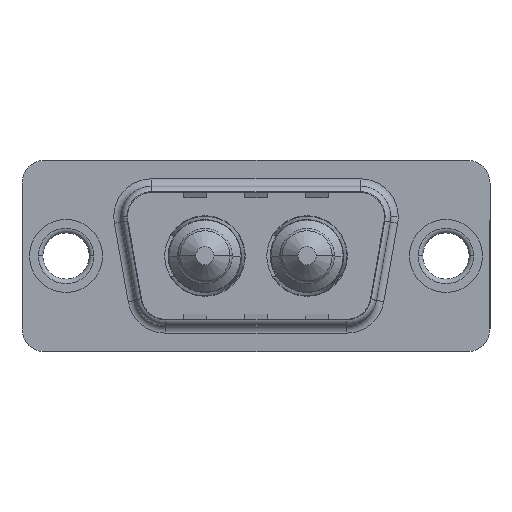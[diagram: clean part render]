
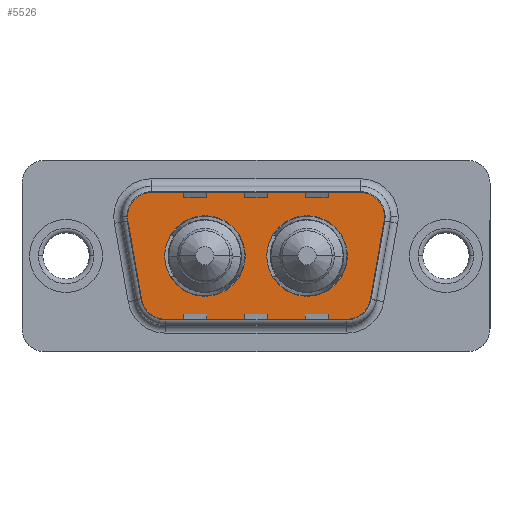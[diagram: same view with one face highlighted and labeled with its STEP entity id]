
A CAD part, top view. The second image highlights one B-rep face of the part: STEP entity #5526.
In plain terms, the highlighted planar face has unit normal (0, 0, 1).
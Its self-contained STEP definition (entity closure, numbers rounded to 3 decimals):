
#212 = CARTESIAN_POINT ( 'NONE',  ( 6.459, -4.9, 0. ) ) ;
#232 = CARTESIAN_POINT ( 'NONE',  ( 18.541, -2.9, 0. ) ) ;
#290 = DIRECTION ( 'NONE',  ( -1., 0., 0. ) ) ;
#355 = AXIS2_PLACEMENT_3D ( 'NONE', #8448, #8273, #8447 ) ;
#385 = VERTEX_POINT ( 'NONE', #918 ) ;
#474 = DIRECTION ( 'NONE',  ( 1., 0., 0. ) ) ;
#530 = VERTEX_POINT ( 'NONE', #7676 ) ;
#533 = CARTESIAN_POINT ( 'NONE',  ( 15.86, 0., 0. ) ) ;
#654 = VERTEX_POINT ( 'NONE', #1199 ) ;
#786 = VERTEX_POINT ( 'NONE', #3515 ) ;
#918 = CARTESIAN_POINT ( 'NONE',  ( 13.21, 0., 0. ) ) ;
#1045 = EDGE_CURVE ( 'NONE', #786, #4447, #5117, .T. ) ;
#1071 = CARTESIAN_POINT ( 'NONE',  ( 5.436, 4.9, 0. ) ) ;
#1079 = DIRECTION ( 'NONE',  ( 1., 0., 0. ) ) ;
#1147 = EDGE_CURVE ( 'NONE', #385, #530, #6631, .T. ) ;
#1199 = CARTESIAN_POINT ( 'NONE',  ( 18.541, -4.9, 0. ) ) ;
#1221 = VERTEX_POINT ( 'NONE', #5766 ) ;
#1385 = VERTEX_POINT ( 'NONE', #1425 ) ;
#1402 = AXIS2_PLACEMENT_3D ( 'NONE', #232, #3843, #3832 ) ;
#1425 = CARTESIAN_POINT ( 'NONE',  ( 6.49, 0., 0. ) ) ;
#1541 = EDGE_CURVE ( 'NONE', #5307, #1221, #9070, .T. ) ;
#1568 = DIRECTION ( 'NONE',  ( 0., 0., 1. ) ) ;
#1749 = DIRECTION ( 'NONE',  ( 0., 0., 1. ) ) ;
#1756 = DIRECTION ( 'NONE',  ( -1., 0., 0. ) ) ;
#1785 = CIRCLE ( 'NONE', #7042, 2.65 ) ;
#1994 = ORIENTED_EDGE ( 'NONE', *, *, #9105, .F. ) ;
#2124 = DIRECTION ( 'NONE',  ( -1., 0., 0. ) ) ;
#2161 = DIRECTION ( 'NONE',  ( 0., 0., 1. ) ) ;
#2173 = CARTESIAN_POINT ( 'NONE',  ( 6.459, -2.9, 0. ) ) ;
#2179 = ORIENTED_EDGE ( 'NONE', *, *, #5018, .T. ) ;
#2181 = DIRECTION ( 'NONE',  ( 0., 0., 1. ) ) ;
#2850 = FACE_BOUND ( 'NONE', #7010, .T. ) ;
#2870 = EDGE_CURVE ( 'NONE', #5521, #654, #6615, .T. ) ;
#3006 = CARTESIAN_POINT ( 'NONE',  ( 21.534, 2.553, 0. ) ) ;
#3131 = CIRCLE ( 'NONE', #4388, 2.65 ) ;
#3275 = DIRECTION ( 'NONE',  ( 1., 0., 0. ) ) ;
#3515 = CARTESIAN_POINT ( 'NONE',  ( 5.436, 4.9, 0. ) ) ;
#3553 = ORIENTED_EDGE ( 'NONE', *, *, #4638, .T. ) ;
#3649 = ORIENTED_EDGE ( 'NONE', *, *, #5430, .F. ) ;
#3773 = CARTESIAN_POINT ( 'NONE',  ( 21.564, 2.9, 0. ) ) ;
#3832 = DIRECTION ( 'NONE',  ( 1., 0., 0. ) ) ;
#3843 = DIRECTION ( 'NONE',  ( 0., 0., 1. ) ) ;
#3860 = VERTEX_POINT ( 'NONE', #8838 ) ;
#3932 = ORIENTED_EDGE ( 'NONE', *, *, #1541, .T. ) ;
#4185 = CARTESIAN_POINT ( 'NONE',  ( 6.459, -4.9, 0. ) ) ;
#4192 = VECTOR ( 'NONE', #290, 1000. ) ;
#4201 = ORIENTED_EDGE ( 'NONE', *, *, #7441, .T. ) ;
#4312 = LINE ( 'NONE', #5502, #8257 ) ;
#4388 = AXIS2_PLACEMENT_3D ( 'NONE', #533, #1568, #1079 ) ;
#4447 = VERTEX_POINT ( 'NONE', #7690 ) ;
#4591 = FACE_OUTER_BOUND ( 'NONE', #4998, .T. ) ;
#4638 = EDGE_CURVE ( 'NONE', #654, #4679, #8320, .T. ) ;
#4679 = VERTEX_POINT ( 'NONE', #7792 ) ;
#4998 = EDGE_LOOP ( 'NONE', ( #3553, #2179, #9634, #3932, #7600, #5657, #4201, #6311, #7351 ) ) ;
#5018 = EDGE_CURVE ( 'NONE', #4679, #9302, #5072, .T. ) ;
#5072 = LINE ( 'NONE', #8224, #6824 ) ;
#5117 = CIRCLE ( 'NONE', #6511, 2. ) ;
#5134 = DIRECTION ( 'NONE',  ( 0., 0., 1. ) ) ;
#5307 = VERTEX_POINT ( 'NONE', #3773 ) ;
#5313 = PLANE ( 'NONE',  #1402 ) ;
#5430 = EDGE_CURVE ( 'NONE', #1385, #7245, #1785, .T. ) ;
#5468 = DIRECTION ( 'NONE',  ( -1., 0., 0. ) ) ;
#5495 = EDGE_CURVE ( 'NONE', #3860, #5521, #6813, .T. ) ;
#5502 = CARTESIAN_POINT ( 'NONE',  ( 3.466, 2.553, 0. ) ) ;
#5521 = VERTEX_POINT ( 'NONE', #212 ) ;
#5526 = ADVANCED_FACE ( 'NONE', ( #6567, #2850, #4591 ), #5313, .T. ) ;
#5551 = CIRCLE ( 'NONE', #6382, 2.65 ) ;
#5575 = DIRECTION ( 'NONE',  ( 0.174, -0.985, 0. ) ) ;
#5657 = ORIENTED_EDGE ( 'NONE', *, *, #1045, .T. ) ;
#5766 = CARTESIAN_POINT ( 'NONE',  ( 19.564, 4.9, 0. ) ) ;
#5957 = CARTESIAN_POINT ( 'NONE',  ( 5.436, 2.9, 0. ) ) ;
#5978 = CARTESIAN_POINT ( 'NONE',  ( 11.79, 0., 0. ) ) ;
#6142 = VECTOR ( 'NONE', #9294, 1000. ) ;
#6144 = AXIS2_PLACEMENT_3D ( 'NONE', #6692, #5134, #5468 ) ;
#6160 = LINE ( 'NONE', #1071, #4192 ) ;
#6220 = EDGE_LOOP ( 'NONE', ( #7129, #7264 ) ) ;
#6272 = CIRCLE ( 'NONE', #8299, 2. ) ;
#6311 = ORIENTED_EDGE ( 'NONE', *, *, #5495, .T. ) ;
#6382 = AXIS2_PLACEMENT_3D ( 'NONE', #6854, #6796, #6789 ) ;
#6511 = AXIS2_PLACEMENT_3D ( 'NONE', #5957, #2181, #3275 ) ;
#6567 = FACE_BOUND ( 'NONE', #6220, .T. ) ;
#6615 = LINE ( 'NONE', #4185, #6142 ) ;
#6631 = CIRCLE ( 'NONE', #355, 2.65 ) ;
#6692 = CARTESIAN_POINT ( 'NONE',  ( 19.564, 2.9, 0. ) ) ;
#6768 = AXIS2_PLACEMENT_3D ( 'NONE', #6964, #6815, #474 ) ;
#6789 = DIRECTION ( 'NONE',  ( 1., 0., 0. ) ) ;
#6796 = DIRECTION ( 'NONE',  ( 0., 0., 1. ) ) ;
#6813 = CIRCLE ( 'NONE', #9046, 2. ) ;
#6815 = DIRECTION ( 'NONE',  ( 0., 0., 1. ) ) ;
#6824 = VECTOR ( 'NONE', #8265, 1000. ) ;
#6854 = CARTESIAN_POINT ( 'NONE',  ( 9.14, 0., 0. ) ) ;
#6964 = CARTESIAN_POINT ( 'NONE',  ( 18.541, -2.9, 0. ) ) ;
#7006 = DIRECTION ( 'NONE',  ( 1., 0., 0. ) ) ;
#7010 = EDGE_LOOP ( 'NONE', ( #1994, #3649 ) ) ;
#7026 = DIRECTION ( 'NONE',  ( 0., 0., 1. ) ) ;
#7032 = CARTESIAN_POINT ( 'NONE',  ( 9.14, 0., 0. ) ) ;
#7042 = AXIS2_PLACEMENT_3D ( 'NONE', #7032, #7026, #7006 ) ;
#7129 = ORIENTED_EDGE ( 'NONE', *, *, #7591, .F. ) ;
#7245 = VERTEX_POINT ( 'NONE', #5978 ) ;
#7264 = ORIENTED_EDGE ( 'NONE', *, *, #1147, .F. ) ;
#7351 = ORIENTED_EDGE ( 'NONE', *, *, #2870, .T. ) ;
#7441 = EDGE_CURVE ( 'NONE', #4447, #3860, #4312, .T. ) ;
#7591 = EDGE_CURVE ( 'NONE', #530, #385, #3131, .T. ) ;
#7600 = ORIENTED_EDGE ( 'NONE', *, *, #7689, .T. ) ;
#7676 = CARTESIAN_POINT ( 'NONE',  ( 18.51, 0., 0. ) ) ;
#7689 = EDGE_CURVE ( 'NONE', #1221, #786, #6160, .T. ) ;
#7690 = CARTESIAN_POINT ( 'NONE',  ( 3.466, 2.553, 0. ) ) ;
#7773 = CARTESIAN_POINT ( 'NONE',  ( 19.564, 2.9, 0. ) ) ;
#7792 = CARTESIAN_POINT ( 'NONE',  ( 20.511, -3.247, 0. ) ) ;
#7969 = EDGE_CURVE ( 'NONE', #9302, #5307, #6272, .T. ) ;
#8224 = CARTESIAN_POINT ( 'NONE',  ( 21.534, 2.553, 0. ) ) ;
#8257 = VECTOR ( 'NONE', #5575, 1000. ) ;
#8265 = DIRECTION ( 'NONE',  ( 0.174, 0.985, 0. ) ) ;
#8273 = DIRECTION ( 'NONE',  ( 0., 0., 1. ) ) ;
#8299 = AXIS2_PLACEMENT_3D ( 'NONE', #7773, #1749, #1756 ) ;
#8320 = CIRCLE ( 'NONE', #6768, 2. ) ;
#8447 = DIRECTION ( 'NONE',  ( 1., 0., 0. ) ) ;
#8448 = CARTESIAN_POINT ( 'NONE',  ( 15.86, 0., 0. ) ) ;
#8838 = CARTESIAN_POINT ( 'NONE',  ( 4.489, -3.247, 0. ) ) ;
#9046 = AXIS2_PLACEMENT_3D ( 'NONE', #2173, #2161, #2124 ) ;
#9070 = CIRCLE ( 'NONE', #6144, 2. ) ;
#9105 = EDGE_CURVE ( 'NONE', #7245, #1385, #5551, .T. ) ;
#9294 = DIRECTION ( 'NONE',  ( 1., 0., 0. ) ) ;
#9302 = VERTEX_POINT ( 'NONE', #3006 ) ;
#9634 = ORIENTED_EDGE ( 'NONE', *, *, #7969, .T. ) ;
